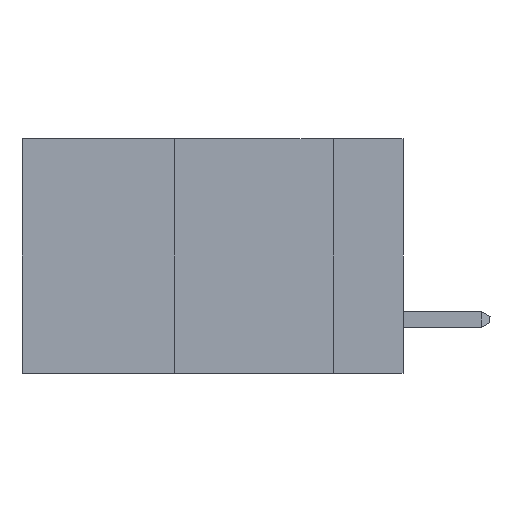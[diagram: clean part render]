
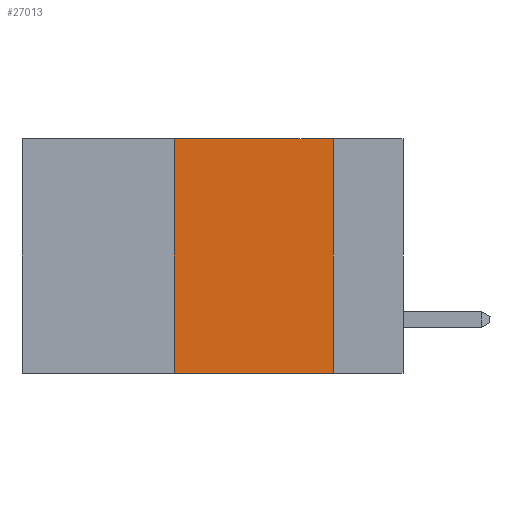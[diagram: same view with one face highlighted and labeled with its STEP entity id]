
A CAD part, left-side view. The second image highlights one B-rep face of the part: STEP entity #27013.
In plain terms, the highlighted planar face has unit normal (-1, 0, 0).
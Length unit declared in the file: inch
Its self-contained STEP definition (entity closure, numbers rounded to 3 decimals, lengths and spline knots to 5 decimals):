
#1544 = LINE ( 'NONE', #30306, #20685 ) ;
#1876 = DIRECTION ( 'NONE',  ( 0., 0., 1. ) ) ;
#1948 = ORIENTED_EDGE ( 'NONE', *, *, #3322, .F. ) ;
#2420 = CARTESIAN_POINT ( 'NONE',  ( 0., 0.6, 0. ) ) ;
#3322 = EDGE_CURVE ( 'NONE', #20194, #8888, #6784, .T. ) ;
#3507 = VERTEX_POINT ( 'NONE', #10689 ) ;
#3757 = DIRECTION ( 'NONE',  ( 0., 0., -1. ) ) ;
#6169 = DIRECTION ( 'NONE',  ( 1., 0., 0. ) ) ;
#6784 = LINE ( 'NONE', #32806, #30208 ) ;
#7123 = ORIENTED_EDGE ( 'NONE', *, *, #33334, .T. ) ;
#8708 = ORIENTED_EDGE ( 'NONE', *, *, #11711, .F. ) ;
#8888 = VERTEX_POINT ( 'NONE', #30141 ) ;
#9207 = DIRECTION ( 'NONE',  ( 0., 0., -1. ) ) ;
#10689 = CARTESIAN_POINT ( 'NONE',  ( 0., 0.36, 0. ) ) ;
#10875 = DIRECTION ( 'NONE',  ( 0., -1., 0. ) ) ;
#11711 = EDGE_CURVE ( 'NONE', #3507, #20194, #12590, .T. ) ;
#12111 = ORIENTED_EDGE ( 'NONE', *, *, #16409, .F. ) ;
#12590 = LINE ( 'NONE', #2420, #31535 ) ;
#15682 = VERTEX_POINT ( 'NONE', #29003 ) ;
#16409 = EDGE_CURVE ( 'NONE', #15682, #3507, #1544, .T. ) ;
#19431 = PLANE ( 'NONE',  #32629 ) ;
#19510 = VECTOR ( 'NONE', #20891, 39.37008 ) ;
#20194 = VERTEX_POINT ( 'NONE', #24248 ) ;
#20547 = LINE ( 'NONE', #23127, #19510 ) ;
#20685 = VECTOR ( 'NONE', #1876, 39.37008 ) ;
#20891 = DIRECTION ( 'NONE',  ( 0., -1., 0. ) ) ;
#23127 = CARTESIAN_POINT ( 'NONE',  ( 0., 0.6, -0.37 ) ) ;
#23266 = EDGE_LOOP ( 'NONE', ( #1948, #8708, #12111, #7123 ) ) ;
#24105 = CARTESIAN_POINT ( 'NONE',  ( 0., 0.6, 0. ) ) ;
#24248 = CARTESIAN_POINT ( 'NONE',  ( 0., 0.11, 0. ) ) ;
#27013 = ADVANCED_FACE ( 'NONE', ( #32682 ), #19431, .F. ) ;
#29003 = CARTESIAN_POINT ( 'NONE',  ( 0., 0.36, -0.37 ) ) ;
#30141 = CARTESIAN_POINT ( 'NONE',  ( 0., 0.11, -0.37 ) ) ;
#30208 = VECTOR ( 'NONE', #9207, 39.37008 ) ;
#30306 = CARTESIAN_POINT ( 'NONE',  ( 0., 0.36, 0. ) ) ;
#31535 = VECTOR ( 'NONE', #10875, 39.37008 ) ;
#32629 = AXIS2_PLACEMENT_3D ( 'NONE', #24105, #6169, #3757 ) ;
#32682 = FACE_OUTER_BOUND ( 'NONE', #23266, .T. ) ;
#32806 = CARTESIAN_POINT ( 'NONE',  ( 0., 0.11, 0. ) ) ;
#33334 = EDGE_CURVE ( 'NONE', #15682, #8888, #20547, .T. ) ;
